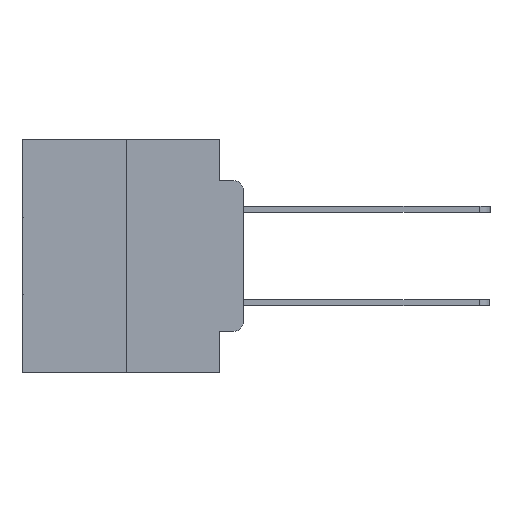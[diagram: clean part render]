
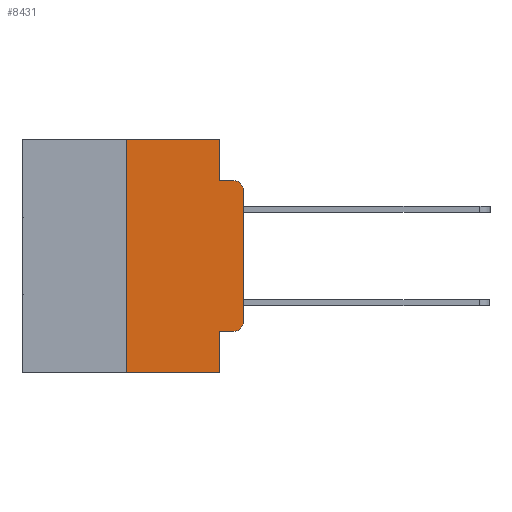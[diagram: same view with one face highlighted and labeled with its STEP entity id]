
A CAD part, left-side view. The second image highlights one B-rep face of the part: STEP entity #8431.
In plain terms, the highlighted planar face has unit normal (-1, 0, 0).
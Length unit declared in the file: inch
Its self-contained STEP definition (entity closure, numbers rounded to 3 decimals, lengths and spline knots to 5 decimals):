
#206 = ORIENTED_EDGE ( 'NONE', *, *, #14908, .T. ) ;
#520 = PLANE ( 'NONE',  #27252 ) ;
#609 = CARTESIAN_POINT ( 'NONE',  ( 0., 0.473, -0.5 ) ) ;
#661 = DIRECTION ( 'NONE',  ( -1., 0., 0. ) ) ;
#916 = VERTEX_POINT ( 'NONE', #27689 ) ;
#1264 = DIRECTION ( 'NONE',  ( 0., 0., -1. ) ) ;
#1758 = DIRECTION ( 'NONE',  ( 0., 0., 1. ) ) ;
#2237 = VERTEX_POINT ( 'NONE', #4692 ) ;
#3091 = ORIENTED_EDGE ( 'NONE', *, *, #27185, .F. ) ;
#3194 = EDGE_CURVE ( 'NONE', #16919, #23888, #26066, .T. ) ;
#3345 = VERTEX_POINT ( 'NONE', #28719 ) ;
#3735 = VERTEX_POINT ( 'NONE', #28164 ) ;
#3806 = ORIENTED_EDGE ( 'NONE', *, *, #21073, .F. ) ;
#3858 = CIRCLE ( 'NONE', #4599, 0.02 ) ;
#4164 = CARTESIAN_POINT ( 'NONE',  ( 0., 0.25, -0.5 ) ) ;
#4599 = AXIS2_PLACEMENT_3D ( 'NONE', #14890, #661, #17190 ) ;
#4692 = CARTESIAN_POINT ( 'NONE',  ( 0., 0.051, -0.4115 ) ) ;
#5005 = VERTEX_POINT ( 'NONE', #23240 ) ;
#5304 = CARTESIAN_POINT ( 'NONE',  ( 0., 0.051, 0. ) ) ;
#5410 = DIRECTION ( 'NONE',  ( 0., 0., -1. ) ) ;
#5976 = ORIENTED_EDGE ( 'NONE', *, *, #3194, .F. ) ;
#7318 = CARTESIAN_POINT ( 'NONE',  ( 0., 0.02, -0.1085 ) ) ;
#7587 = LINE ( 'NONE', #5304, #19325 ) ;
#7709 = DIRECTION ( 'NONE',  ( 0., 0., -1. ) ) ;
#7742 = ORIENTED_EDGE ( 'NONE', *, *, #27142, .F. ) ;
#8431 = ADVANCED_FACE ( 'NONE', ( #10157 ), #520, .F. ) ;
#9417 = ORIENTED_EDGE ( 'NONE', *, *, #14333, .T. ) ;
#9520 = EDGE_CURVE ( 'NONE', #3345, #23888, #27432, .T. ) ;
#9677 = DIRECTION ( 'NONE',  ( 0., 0., -1. ) ) ;
#10157 = FACE_OUTER_BOUND ( 'NONE', #19177, .T. ) ;
#10161 = DIRECTION ( 'NONE',  ( 0., -1., 0. ) ) ;
#10323 = CARTESIAN_POINT ( 'NONE',  ( 0., 0., 0. ) ) ;
#10856 = VECTOR ( 'NONE', #28234, 39.37008 ) ;
#10920 = EDGE_CURVE ( 'NONE', #21213, #916, #22023, .T. ) ;
#12995 = ORIENTED_EDGE ( 'NONE', *, *, #9520, .T. ) ;
#13125 = CARTESIAN_POINT ( 'NONE',  ( 0., 0.051, 0. ) ) ;
#13207 = VECTOR ( 'NONE', #17424, 39.37008 ) ;
#13607 = CARTESIAN_POINT ( 'NONE',  ( 0., 0.25, 0. ) ) ;
#14333 = EDGE_CURVE ( 'NONE', #16317, #3345, #19358, .T. ) ;
#14741 = CARTESIAN_POINT ( 'NONE',  ( 0., 0.051, -0.0885 ) ) ;
#14890 = CARTESIAN_POINT ( 'NONE',  ( 0., 0.02, -0.3915 ) ) ;
#14908 = EDGE_CURVE ( 'NONE', #3735, #16317, #3858, .T. ) ;
#14946 = CARTESIAN_POINT ( 'NONE',  ( 0., 0.02, -0.0885 ) ) ;
#15515 = CARTESIAN_POINT ( 'NONE',  ( 0., 0.25, 0. ) ) ;
#15615 = CARTESIAN_POINT ( 'NONE',  ( 0., 0., -0.3915 ) ) ;
#16317 = VERTEX_POINT ( 'NONE', #15615 ) ;
#16765 = DIRECTION ( 'NONE',  ( 0., -1., 0. ) ) ;
#16919 = VERTEX_POINT ( 'NONE', #17527 ) ;
#17163 = CARTESIAN_POINT ( 'NONE',  ( 0., 0.473, 0. ) ) ;
#17164 = CARTESIAN_POINT ( 'NONE',  ( 0., 0.473, 0. ) ) ;
#17190 = DIRECTION ( 'NONE',  ( 0., 0., -1. ) ) ;
#17424 = DIRECTION ( 'NONE',  ( 0., 0., 1. ) ) ;
#17482 = LINE ( 'NONE', #13125, #22144 ) ;
#17527 = CARTESIAN_POINT ( 'NONE',  ( 0., 0.051, -0.0885 ) ) ;
#17602 = LINE ( 'NONE', #13607, #29671 ) ;
#17984 = EDGE_CURVE ( 'NONE', #2237, #3735, #25181, .T. ) ;
#18890 = ORIENTED_EDGE ( 'NONE', *, *, #10920, .T. ) ;
#19122 = VECTOR ( 'NONE', #16765, 39.37008 ) ;
#19177 = EDGE_LOOP ( 'NONE', ( #9417, #12995, #5976, #7742, #3091, #20366, #18890, #3806, #26921, #206 ) ) ;
#19325 = VECTOR ( 'NONE', #7709, 39.37008 ) ;
#19358 = LINE ( 'NONE', #10323, #13207 ) ;
#19488 = DIRECTION ( 'NONE',  ( 0., -1., 0. ) ) ;
#19500 = DIRECTION ( 'NONE',  ( 1., 0., 0. ) ) ;
#20366 = ORIENTED_EDGE ( 'NONE', *, *, #25621, .F. ) ;
#20500 = VERTEX_POINT ( 'NONE', #15515 ) ;
#21073 = EDGE_CURVE ( 'NONE', #2237, #916, #17482, .T. ) ;
#21213 = VERTEX_POINT ( 'NONE', #4164 ) ;
#21301 = CARTESIAN_POINT ( 'NONE',  ( 0., 0.051, -0.4115 ) ) ;
#22023 = LINE ( 'NONE', #609, #22724 ) ;
#22144 = VECTOR ( 'NONE', #1264, 39.37008 ) ;
#22724 = VECTOR ( 'NONE', #19488, 39.37008 ) ;
#23240 = CARTESIAN_POINT ( 'NONE',  ( 0., 0.051, 0. ) ) ;
#23618 = DIRECTION ( 'NONE',  ( -1., 0., 0. ) ) ;
#23888 = VERTEX_POINT ( 'NONE', #14946 ) ;
#23958 = VECTOR ( 'NONE', #10161, 39.37008 ) ;
#25181 = LINE ( 'NONE', #21301, #19122 ) ;
#25621 = EDGE_CURVE ( 'NONE', #21213, #20500, #17602, .T. ) ;
#26066 = LINE ( 'NONE', #14741, #10856 ) ;
#26921 = ORIENTED_EDGE ( 'NONE', *, *, #17984, .T. ) ;
#27142 = EDGE_CURVE ( 'NONE', #5005, #16919, #7587, .T. ) ;
#27185 = EDGE_CURVE ( 'NONE', #20500, #5005, #29910, .T. ) ;
#27252 = AXIS2_PLACEMENT_3D ( 'NONE', #17164, #19500, #5410 ) ;
#27432 = CIRCLE ( 'NONE', #28590, 0.02 ) ;
#27689 = CARTESIAN_POINT ( 'NONE',  ( 0., 0.051, -0.5 ) ) ;
#28164 = CARTESIAN_POINT ( 'NONE',  ( 0., 0.02, -0.4115 ) ) ;
#28234 = DIRECTION ( 'NONE',  ( 0., -1., 0. ) ) ;
#28590 = AXIS2_PLACEMENT_3D ( 'NONE', #7318, #23618, #9677 ) ;
#28719 = CARTESIAN_POINT ( 'NONE',  ( 0., 0., -0.1085 ) ) ;
#29671 = VECTOR ( 'NONE', #1758, 39.37008 ) ;
#29910 = LINE ( 'NONE', #17163, #23958 ) ;
